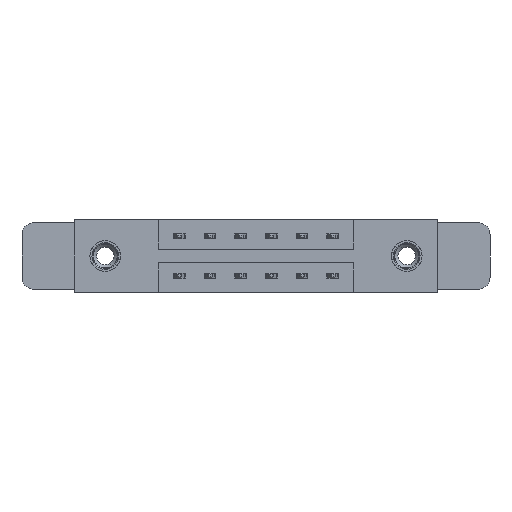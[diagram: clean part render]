
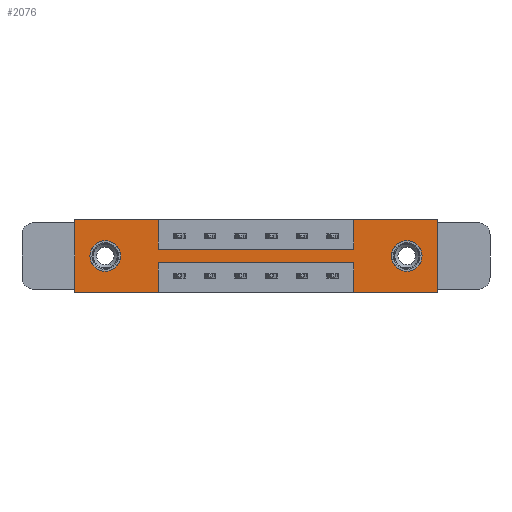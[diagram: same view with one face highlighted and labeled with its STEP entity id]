
A CAD part, front view. The second image highlights one B-rep face of the part: STEP entity #2076.
In plain terms, the highlighted planar face has unit normal (0, -1, 0).
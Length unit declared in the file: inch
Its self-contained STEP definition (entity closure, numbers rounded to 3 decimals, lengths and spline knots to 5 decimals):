
#3 = CARTESIAN_POINT ( 'NONE',  ( 0.155, 0., -0.185 ) ) ;
#127 = DIRECTION ( 'NONE',  ( 0., 0., 1. ) ) ;
#200 = DIRECTION ( 'NONE',  ( 0., 0., -1. ) ) ;
#252 = DIRECTION ( 'NONE',  ( 0., 0., 1. ) ) ;
#463 = EDGE_LOOP ( 'NONE', ( #855, #3682, #8444, #1142, #5564, #2737, #7075, #11373, #4215, #1661, #5109, #5982 ) ) ;
#848 = ORIENTED_EDGE ( 'NONE', *, *, #1039, .T. ) ;
#851 = AXIS2_PLACEMENT_3D ( 'NONE', #9424, #10364, #200 ) ;
#855 = ORIENTED_EDGE ( 'NONE', *, *, #9074, .F. ) ;
#874 = CARTESIAN_POINT ( 'NONE',  ( 0., 0., 0. ) ) ;
#1019 = CIRCLE ( 'NONE', #10274, 0.078 ) ;
#1039 = EDGE_CURVE ( 'NONE', #3126, #4888, #8033, .T. ) ;
#1141 = DIRECTION ( 'NONE',  ( 0., 0., 1. ) ) ;
#1142 = ORIENTED_EDGE ( 'NONE', *, *, #11437, .F. ) ;
#1150 = EDGE_CURVE ( 'NONE', #2456, #6904, #5280, .T. ) ;
#1238 = ORIENTED_EDGE ( 'NONE', *, *, #8496, .T. ) ;
#1293 = CARTESIAN_POINT ( 'NONE',  ( 0., 0., 0. ) ) ;
#1319 = AXIS2_PLACEMENT_3D ( 'NONE', #3, #3720, #6578 ) ;
#1327 = VERTEX_POINT ( 'NONE', #9877 ) ;
#1368 = VERTEX_POINT ( 'NONE', #6158 ) ;
#1395 = LINE ( 'NONE', #3456, #3553 ) ;
#1411 = EDGE_CURVE ( 'NONE', #1327, #6873, #1395, .T. ) ;
#1518 = VECTOR ( 'NONE', #6899, 39.37008 ) ;
#1661 = ORIENTED_EDGE ( 'NONE', *, *, #1411, .F. ) ;
#1737 = EDGE_CURVE ( 'NONE', #10361, #6912, #5703, .T. ) ;
#1793 = DIRECTION ( 'NONE',  ( 1., 0., 0. ) ) ;
#2076 = ADVANCED_FACE ( 'NONE', ( #2667, #7283, #4820 ), #7676, .T. ) ;
#2456 = VERTEX_POINT ( 'NONE', #9382 ) ;
#2602 = DIRECTION ( 'NONE',  ( 1., 0., 0. ) ) ;
#2606 = VECTOR ( 'NONE', #5812, 39.37008 ) ;
#2667 = FACE_BOUND ( 'NONE', #6843, .T. ) ;
#2737 = ORIENTED_EDGE ( 'NONE', *, *, #11303, .F. ) ;
#2932 = LINE ( 'NONE', #7100, #10021 ) ;
#3058 = DIRECTION ( 'NONE',  ( -1., 0., 0. ) ) ;
#3126 = VERTEX_POINT ( 'NONE', #5945 ) ;
#3260 = CARTESIAN_POINT ( 'NONE',  ( 1.417, 0., -0.22 ) ) ;
#3321 = DIRECTION ( 'NONE',  ( 0., 0., -1. ) ) ;
#3456 = CARTESIAN_POINT ( 'NONE',  ( 0., 0., 0. ) ) ;
#3547 = VERTEX_POINT ( 'NONE', #8561 ) ;
#3553 = VECTOR ( 'NONE', #6225, 39.37008 ) ;
#3606 = VERTEX_POINT ( 'NONE', #9415 ) ;
#3682 = ORIENTED_EDGE ( 'NONE', *, *, #10107, .F. ) ;
#3720 = DIRECTION ( 'NONE',  ( 0., 1., 0. ) ) ;
#3780 = VECTOR ( 'NONE', #1793, 39.37008 ) ;
#3906 = CARTESIAN_POINT ( 'NONE',  ( 0.425, 0., -0.22 ) ) ;
#3918 = CARTESIAN_POINT ( 'NONE',  ( 1.687, 0., -0.263 ) ) ;
#4055 = CARTESIAN_POINT ( 'NONE',  ( 1.417, 0., 0. ) ) ;
#4170 = AXIS2_PLACEMENT_3D ( 'NONE', #8060, #8944, #9946 ) ;
#4215 = ORIENTED_EDGE ( 'NONE', *, *, #8890, .F. ) ;
#4332 = LINE ( 'NONE', #10438, #2606 ) ;
#4464 = AXIS2_PLACEMENT_3D ( 'NONE', #11222, #5662, #127 ) ;
#4820 = FACE_OUTER_BOUND ( 'NONE', #463, .T. ) ;
#4844 = CARTESIAN_POINT ( 'NONE',  ( 0.425, 0., 0. ) ) ;
#4853 = VECTOR ( 'NONE', #252, 39.37008 ) ;
#4888 = VERTEX_POINT ( 'NONE', #10346 ) ;
#5013 = DIRECTION ( 'NONE',  ( -1., 0., 0. ) ) ;
#5109 = ORIENTED_EDGE ( 'NONE', *, *, #11042, .F. ) ;
#5232 = VERTEX_POINT ( 'NONE', #7967 ) ;
#5234 = VECTOR ( 'NONE', #3058, 39.37008 ) ;
#5280 = LINE ( 'NONE', #5792, #4853 ) ;
#5564 = ORIENTED_EDGE ( 'NONE', *, *, #11129, .F. ) ;
#5662 = DIRECTION ( 'NONE',  ( 0., 1., 0. ) ) ;
#5703 = LINE ( 'NONE', #8809, #1518 ) ;
#5791 = LINE ( 'NONE', #4055, #9129 ) ;
#5792 = CARTESIAN_POINT ( 'NONE',  ( 1.417, 0., -0.37 ) ) ;
#5812 = DIRECTION ( 'NONE',  ( 0., 0., -1. ) ) ;
#5945 = CARTESIAN_POINT ( 'NONE',  ( 0.155, 0., -0.107 ) ) ;
#5982 = ORIENTED_EDGE ( 'NONE', *, *, #1737, .F. ) ;
#6158 = CARTESIAN_POINT ( 'NONE',  ( 0.425, 0., -0.22 ) ) ;
#6225 = DIRECTION ( 'NONE',  ( 1., 0., 0. ) ) ;
#6245 = LINE ( 'NONE', #874, #3780 ) ;
#6333 = LINE ( 'NONE', #9023, #7633 ) ;
#6351 = VECTOR ( 'NONE', #8358, 39.37008 ) ;
#6578 = DIRECTION ( 'NONE',  ( 0., 0., 1. ) ) ;
#6580 = CARTESIAN_POINT ( 'NONE',  ( 0.425, 0., -0.15 ) ) ;
#6843 = EDGE_LOOP ( 'NONE', ( #7442, #1238 ) ) ;
#6873 = VERTEX_POINT ( 'NONE', #10121 ) ;
#6884 = DIRECTION ( 'NONE',  ( 0., 0., -1. ) ) ;
#6899 = DIRECTION ( 'NONE',  ( -1., 0., 0. ) ) ;
#6904 = VERTEX_POINT ( 'NONE', #3260 ) ;
#6912 = VERTEX_POINT ( 'NONE', #11557 ) ;
#6978 = LINE ( 'NONE', #9485, #5234 ) ;
#7048 = CARTESIAN_POINT ( 'NONE',  ( 1.687, 0., -0.185 ) ) ;
#7075 = ORIENTED_EDGE ( 'NONE', *, *, #8431, .F. ) ;
#7100 = CARTESIAN_POINT ( 'NONE',  ( 1.842, 0., 0. ) ) ;
#7171 = EDGE_LOOP ( 'NONE', ( #848, #10668 ) ) ;
#7283 = FACE_BOUND ( 'NONE', #7171, .T. ) ;
#7442 = ORIENTED_EDGE ( 'NONE', *, *, #10292, .T. ) ;
#7633 = VECTOR ( 'NONE', #2602, 39.37008 ) ;
#7676 = PLANE ( 'NONE',  #851 ) ;
#7967 = CARTESIAN_POINT ( 'NONE',  ( 1.842, 0., 0. ) ) ;
#8033 = CIRCLE ( 'NONE', #4464, 0.078 ) ;
#8051 = LINE ( 'NONE', #3906, #10692 ) ;
#8060 = CARTESIAN_POINT ( 'NONE',  ( 1.687, 0., -0.185 ) ) ;
#8214 = VERTEX_POINT ( 'NONE', #6580 ) ;
#8358 = DIRECTION ( 'NONE',  ( 0., 0., -1. ) ) ;
#8391 = VERTEX_POINT ( 'NONE', #3918 ) ;
#8431 = EDGE_CURVE ( 'NONE', #11094, #9992, #5791, .T. ) ;
#8444 = ORIENTED_EDGE ( 'NONE', *, *, #1150, .F. ) ;
#8496 = EDGE_CURVE ( 'NONE', #8391, #3606, #1019, .T. ) ;
#8561 = CARTESIAN_POINT ( 'NONE',  ( 1.842, 0., -0.37 ) ) ;
#8712 = DIRECTION ( 'NONE',  ( 0., 0., 1. ) ) ;
#8809 = CARTESIAN_POINT ( 'NONE',  ( 0., 0., -0.37 ) ) ;
#8890 = EDGE_CURVE ( 'NONE', #6873, #8214, #9993, .T. ) ;
#8944 = DIRECTION ( 'NONE',  ( 0., 1., 0. ) ) ;
#9023 = CARTESIAN_POINT ( 'NONE',  ( 0.425, 0., -0.15 ) ) ;
#9074 = EDGE_CURVE ( 'NONE', #1368, #10361, #4332, .T. ) ;
#9129 = VECTOR ( 'NONE', #1141, 39.37008 ) ;
#9382 = CARTESIAN_POINT ( 'NONE',  ( 1.417, 0., -0.37 ) ) ;
#9415 = CARTESIAN_POINT ( 'NONE',  ( 1.687, 0., -0.107 ) ) ;
#9424 = CARTESIAN_POINT ( 'NONE',  ( 0., 0., -0.37 ) ) ;
#9485 = CARTESIAN_POINT ( 'NONE',  ( 0., 0., -0.37 ) ) ;
#9549 = CARTESIAN_POINT ( 'NONE',  ( 1.417, 0., 0. ) ) ;
#9751 = EDGE_CURVE ( 'NONE', #8214, #11094, #6333, .T. ) ;
#9877 = CARTESIAN_POINT ( 'NONE',  ( 0., 0., 0. ) ) ;
#9946 = DIRECTION ( 'NONE',  ( 0., 0., -1. ) ) ;
#9992 = VERTEX_POINT ( 'NONE', #9549 ) ;
#9993 = LINE ( 'NONE', #4844, #6351 ) ;
#10021 = VECTOR ( 'NONE', #3321, 39.37008 ) ;
#10107 = EDGE_CURVE ( 'NONE', #6904, #1368, #8051, .T. ) ;
#10121 = CARTESIAN_POINT ( 'NONE',  ( 0.425, 0., 0. ) ) ;
#10155 = CIRCLE ( 'NONE', #1319, 0.078 ) ;
#10274 = AXIS2_PLACEMENT_3D ( 'NONE', #7048, #10660, #6884 ) ;
#10292 = EDGE_CURVE ( 'NONE', #3606, #8391, #11414, .T. ) ;
#10312 = VECTOR ( 'NONE', #8712, 39.37008 ) ;
#10346 = CARTESIAN_POINT ( 'NONE',  ( 0.155, 0., -0.263 ) ) ;
#10361 = VERTEX_POINT ( 'NONE', #11862 ) ;
#10364 = DIRECTION ( 'NONE',  ( 0., -1., 0. ) ) ;
#10438 = CARTESIAN_POINT ( 'NONE',  ( 0.425, 0., -0.37 ) ) ;
#10660 = DIRECTION ( 'NONE',  ( 0., 1., 0. ) ) ;
#10668 = ORIENTED_EDGE ( 'NONE', *, *, #11926, .T. ) ;
#10692 = VECTOR ( 'NONE', #5013, 39.37008 ) ;
#10839 = CARTESIAN_POINT ( 'NONE',  ( 1.417, 0., -0.15 ) ) ;
#11042 = EDGE_CURVE ( 'NONE', #6912, #1327, #11760, .T. ) ;
#11094 = VERTEX_POINT ( 'NONE', #10839 ) ;
#11129 = EDGE_CURVE ( 'NONE', #5232, #3547, #2932, .T. ) ;
#11222 = CARTESIAN_POINT ( 'NONE',  ( 0.155, 0., -0.185 ) ) ;
#11303 = EDGE_CURVE ( 'NONE', #9992, #5232, #6245, .T. ) ;
#11373 = ORIENTED_EDGE ( 'NONE', *, *, #9751, .F. ) ;
#11414 = CIRCLE ( 'NONE', #4170, 0.078 ) ;
#11437 = EDGE_CURVE ( 'NONE', #3547, #2456, #6978, .T. ) ;
#11557 = CARTESIAN_POINT ( 'NONE',  ( 0., 0., -0.37 ) ) ;
#11760 = LINE ( 'NONE', #1293, #10312 ) ;
#11862 = CARTESIAN_POINT ( 'NONE',  ( 0.425, 0., -0.37 ) ) ;
#11926 = EDGE_CURVE ( 'NONE', #4888, #3126, #10155, .T. ) ;
